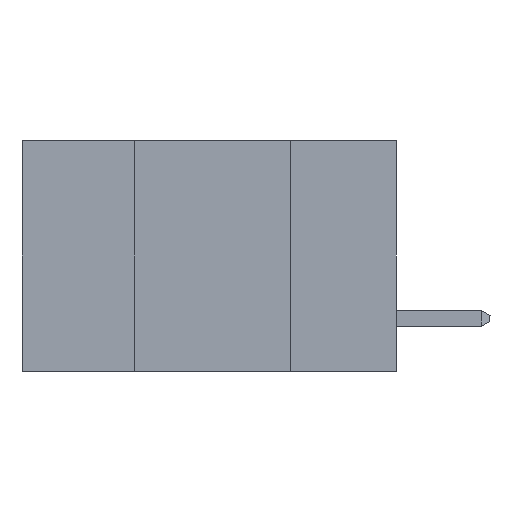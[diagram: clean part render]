
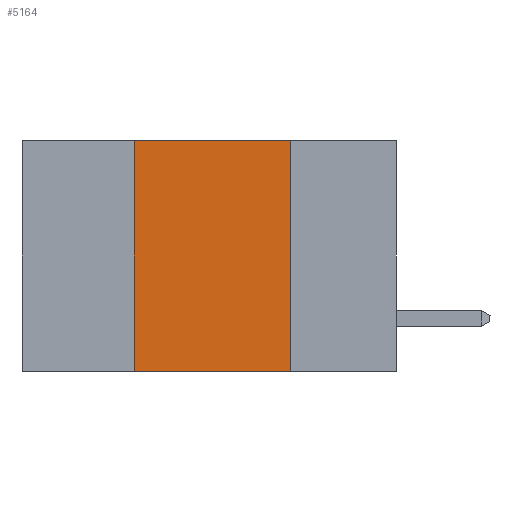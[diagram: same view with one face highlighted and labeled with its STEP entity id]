
A CAD part, left-side view. The second image highlights one B-rep face of the part: STEP entity #5164.
In plain terms, the highlighted planar face has unit normal (-1, 0, 0).
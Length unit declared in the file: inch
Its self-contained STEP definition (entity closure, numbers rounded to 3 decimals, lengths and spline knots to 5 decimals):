
#746 = VECTOR ( 'NONE', #10702, 39.37008 ) ;
#958 = PLANE ( 'NONE',  #7879 ) ;
#1180 = VECTOR ( 'NONE', #1746, 39.37008 ) ;
#1189 = LINE ( 'NONE', #9184, #1419 ) ;
#1419 = VECTOR ( 'NONE', #4919, 39.37008 ) ;
#1616 = VERTEX_POINT ( 'NONE', #3030 ) ;
#1746 = DIRECTION ( 'NONE',  ( 0., 0., -1. ) ) ;
#1819 = CARTESIAN_POINT ( 'NONE',  ( 0., 0.6, 0. ) ) ;
#2178 = EDGE_CURVE ( 'NONE', #7211, #1616, #9741, .T. ) ;
#2598 = DIRECTION ( 'NONE',  ( 0., -1., 0. ) ) ;
#2950 = ORIENTED_EDGE ( 'NONE', *, *, #2178, .F. ) ;
#3030 = CARTESIAN_POINT ( 'NONE',  ( 0., 0.17, -0.37 ) ) ;
#3141 = DIRECTION ( 'NONE',  ( 0., 0., -1. ) ) ;
#3342 = ORIENTED_EDGE ( 'NONE', *, *, #6121, .F. ) ;
#3790 = VERTEX_POINT ( 'NONE', #3863 ) ;
#3863 = CARTESIAN_POINT ( 'NONE',  ( 0., 0.42, -0.37 ) ) ;
#3904 = CARTESIAN_POINT ( 'NONE',  ( 0., 0.42, 0. ) ) ;
#4081 = CARTESIAN_POINT ( 'NONE',  ( 0., 0.42, 0. ) ) ;
#4170 = FACE_OUTER_BOUND ( 'NONE', #4269, .T. ) ;
#4269 = EDGE_LOOP ( 'NONE', ( #2950, #3342, #10322, #8119 ) ) ;
#4324 = EDGE_CURVE ( 'NONE', #3790, #1616, #1189, .T. ) ;
#4408 = DIRECTION ( 'NONE',  ( 1., 0., 0. ) ) ;
#4919 = DIRECTION ( 'NONE',  ( 0., -1., 0. ) ) ;
#5164 = ADVANCED_FACE ( 'NONE', ( #4170 ), #958, .F. ) ;
#5236 = VERTEX_POINT ( 'NONE', #4081 ) ;
#6121 = EDGE_CURVE ( 'NONE', #5236, #7211, #9352, .T. ) ;
#7211 = VERTEX_POINT ( 'NONE', #7391 ) ;
#7391 = CARTESIAN_POINT ( 'NONE',  ( 0., 0.17, 0. ) ) ;
#7879 = AXIS2_PLACEMENT_3D ( 'NONE', #1819, #4408, #3141 ) ;
#8119 = ORIENTED_EDGE ( 'NONE', *, *, #4324, .T. ) ;
#8543 = CARTESIAN_POINT ( 'NONE',  ( 0., 0.6, 0. ) ) ;
#8625 = CARTESIAN_POINT ( 'NONE',  ( 0., 0.17, 0. ) ) ;
#9184 = CARTESIAN_POINT ( 'NONE',  ( 0., 0.6, -0.37 ) ) ;
#9352 = LINE ( 'NONE', #8543, #10685 ) ;
#9583 = LINE ( 'NONE', #3904, #746 ) ;
#9741 = LINE ( 'NONE', #8625, #1180 ) ;
#10322 = ORIENTED_EDGE ( 'NONE', *, *, #10882, .F. ) ;
#10685 = VECTOR ( 'NONE', #2598, 39.37008 ) ;
#10702 = DIRECTION ( 'NONE',  ( 0., 0., 1. ) ) ;
#10882 = EDGE_CURVE ( 'NONE', #3790, #5236, #9583, .T. ) ;
